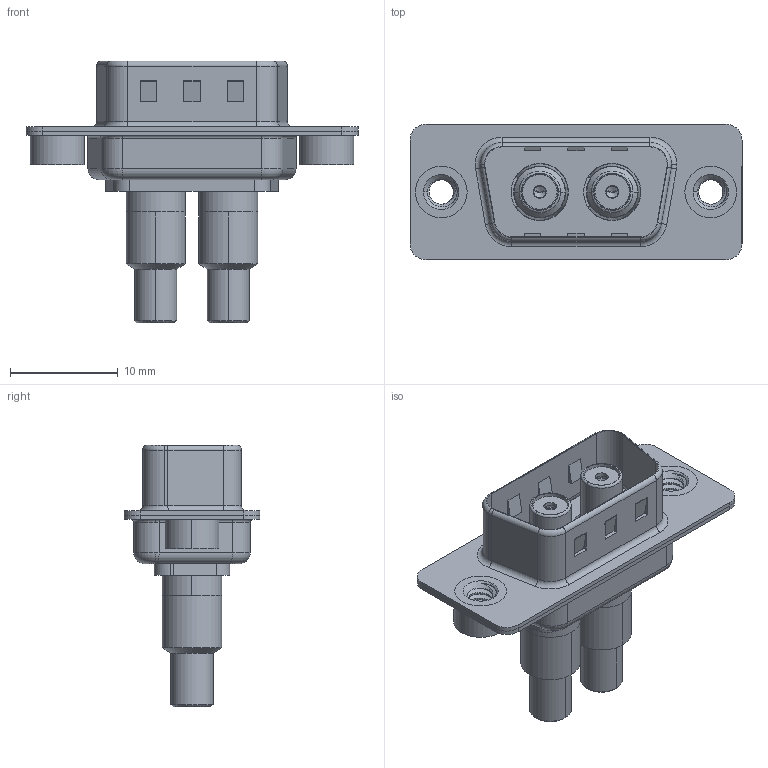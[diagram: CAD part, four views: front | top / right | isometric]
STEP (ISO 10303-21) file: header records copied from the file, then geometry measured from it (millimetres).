
FILE_DESCRIPTION (( 'STEP AP203' ), '1' );
FILE_NAME ('627-2W2-622-5T2.STEP', '2019-05-23T21:27:09', ( '' ), ( '' ), 'SwSTEP 2.0', 'SolidWorks 2016', '' );
FILE_SCHEMA (( 'CONFIG_CONTROL_DESIGN' ));
Length unit declared in the file: millimetre
Products named in the file (12): 627Combo Shell Rear_09 Contacts; 627Combo Shell Front_09 Contacts; 627Combo Threaded Rivet_2; Socket_Solder Cup; Co-Ax Jack_Solder Cup Tail; Solder Cover; Insulator Socket; Co-Ax Jack Assy_SC; Insulator Socket 2; 627-2W2-622-5T2; Locking Collar; 627Combo Housing_2W2
Assembly tree (13 placements, depth 3):
  627-2W2-622-5T2
    627Combo Housing_2W2
    627Combo Shell Rear_09 Contacts
    627Combo Shell Front_09 Contacts
    627Combo Threaded Rivet_2  x2
    Co-Ax Jack Assy_SC  x2
      Co-Ax Jack_Solder Cup Tail
      Insulator Socket
      Insulator Socket 2
      Locking Collar
      Socket_Solder Cup
      Solder Cover
Bounding box: 30.8 x 12.6 x 24.3 mm (x, y, z)
Volume: 1569.1 mm3; surface area: 5263.5 mm2
Topology: 17 solids, 17 shells, 564 faces, 1335 edges, 826 vertices
Faces by surface type: cylinder 257, plane 187, torus 58, cone 52, bspline 10
Entity records: 14706 total; most frequent: CARTESIAN_POINT 3660, DIRECTION 2177, ORIENTED_EDGE 1942, EDGE_CURVE 971, AXIS2_PLACEMENT_3D 849, VERTEX_POINT 606, LINE 479, VECTOR 479
